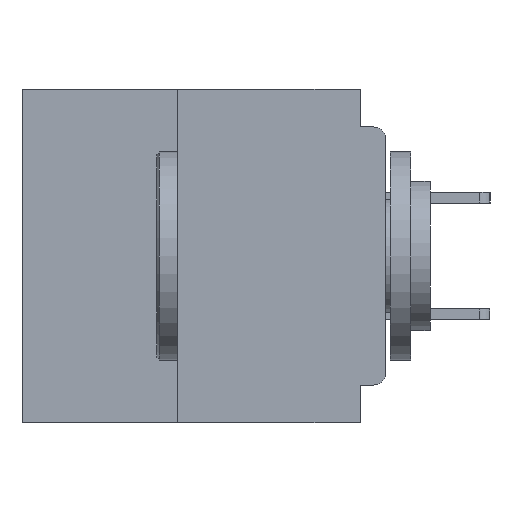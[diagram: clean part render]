
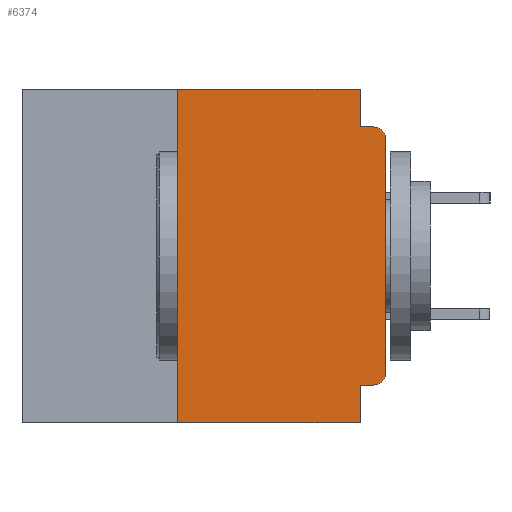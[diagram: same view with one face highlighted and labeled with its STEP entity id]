
A CAD part, left-side view. The second image highlights one B-rep face of the part: STEP entity #6374.
In plain terms, the highlighted planar face has unit normal (-1, 0, 0).
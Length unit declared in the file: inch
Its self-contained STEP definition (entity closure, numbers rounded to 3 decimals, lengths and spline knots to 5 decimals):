
#128 = VECTOR ( 'NONE', #31256, 39.37008 ) ;
#284 = DIRECTION ( 'NONE',  ( -1., 0., 0. ) ) ;
#334 = CARTESIAN_POINT ( 'NONE',  ( 0., 0.031, 0. ) ) ;
#665 = AXIS2_PLACEMENT_3D ( 'NONE', #21856, #284, #25495 ) ;
#1290 = LINE ( 'NONE', #27664, #128 ) ;
#1384 = CIRCLE ( 'NONE', #16615, 0.015 ) ;
#2345 = VERTEX_POINT ( 'NONE', #30027 ) ;
#4031 = LINE ( 'NONE', #44875, #41101 ) ;
#4156 = VERTEX_POINT ( 'NONE', #334 ) ;
#4670 = VECTOR ( 'NONE', #10521, 39.37008 ) ;
#4908 = ORIENTED_EDGE ( 'NONE', *, *, #34543, .T. ) ;
#6158 = VECTOR ( 'NONE', #43915, 39.37008 ) ;
#6374 = ADVANCED_FACE ( 'NONE', ( #24311 ), #21047, .F. ) ;
#6766 = CARTESIAN_POINT ( 'NONE',  ( 0., 0.437, 0. ) ) ;
#7662 = CARTESIAN_POINT ( 'NONE',  ( 0., 0.031, -0.045 ) ) ;
#8150 = EDGE_CURVE ( 'NONE', #38458, #2345, #15741, .T. ) ;
#8468 = CARTESIAN_POINT ( 'NONE',  ( 0., 0.437, -0.4 ) ) ;
#9410 = ORIENTED_EDGE ( 'NONE', *, *, #27634, .T. ) ;
#9823 = VERTEX_POINT ( 'NONE', #33928 ) ;
#10389 = DIRECTION ( 'NONE',  ( 1., 0., 0. ) ) ;
#10521 = DIRECTION ( 'NONE',  ( 0., 0., -1. ) ) ;
#11559 = EDGE_LOOP ( 'NONE', ( #4908, #29991, #24010, #18927, #19372, #18607, #9410, #14994, #15608, #34987 ) ) ;
#11772 = AXIS2_PLACEMENT_3D ( 'NONE', #6766, #10389, #35493 ) ;
#12457 = CARTESIAN_POINT ( 'NONE',  ( 0., 0., -0.06 ) ) ;
#12467 = VERTEX_POINT ( 'NONE', #14058 ) ;
#12930 = EDGE_CURVE ( 'NONE', #43955, #12467, #1290, .T. ) ;
#12963 = DIRECTION ( 'NONE',  ( -1., 0., 0. ) ) ;
#13313 = DIRECTION ( 'NONE',  ( 0., 0., 1. ) ) ;
#14058 = CARTESIAN_POINT ( 'NONE',  ( 0., 0.25, 0. ) ) ;
#14141 = CARTESIAN_POINT ( 'NONE',  ( 0., 0.031, -0.4 ) ) ;
#14639 = EDGE_CURVE ( 'NONE', #4156, #38458, #4031, .T. ) ;
#14994 = ORIENTED_EDGE ( 'NONE', *, *, #24135, .F. ) ;
#15608 = ORIENTED_EDGE ( 'NONE', *, *, #29951, .F. ) ;
#15741 = LINE ( 'NONE', #45934, #23008 ) ;
#16615 = AXIS2_PLACEMENT_3D ( 'NONE', #34432, #12963, #38024 ) ;
#18607 = ORIENTED_EDGE ( 'NONE', *, *, #12930, .F. ) ;
#18927 = ORIENTED_EDGE ( 'NONE', *, *, #14639, .F. ) ;
#19293 = DIRECTION ( 'NONE',  ( 0., -1., 0. ) ) ;
#19372 = ORIENTED_EDGE ( 'NONE', *, *, #29655, .F. ) ;
#21047 = PLANE ( 'NONE',  #11772 ) ;
#21856 = CARTESIAN_POINT ( 'NONE',  ( 0., 0.015, -0.06 ) ) ;
#22746 = VERTEX_POINT ( 'NONE', #37726 ) ;
#22804 = EDGE_CURVE ( 'NONE', #43268, #9823, #1384, .T. ) ;
#23008 = VECTOR ( 'NONE', #28121, 39.37008 ) ;
#23745 = CARTESIAN_POINT ( 'NONE',  ( 0., 0.437, 0. ) ) ;
#23801 = LINE ( 'NONE', #14141, #4670 ) ;
#24010 = ORIENTED_EDGE ( 'NONE', *, *, #8150, .F. ) ;
#24135 = EDGE_CURVE ( 'NONE', #38394, #22746, #23801, .T. ) ;
#24311 = FACE_OUTER_BOUND ( 'NONE', #11559, .T. ) ;
#25262 = LINE ( 'NONE', #33288, #6158 ) ;
#25495 = DIRECTION ( 'NONE',  ( 0., 0., -1. ) ) ;
#27097 = CARTESIAN_POINT ( 'NONE',  ( 0., 0.25, -0.4 ) ) ;
#27634 = EDGE_CURVE ( 'NONE', #43955, #22746, #39466, .T. ) ;
#27664 = CARTESIAN_POINT ( 'NONE',  ( 0., 0.25, -0.4 ) ) ;
#27748 = CARTESIAN_POINT ( 'NONE',  ( 0., 0., 0. ) ) ;
#28121 = DIRECTION ( 'NONE',  ( 0., -1., 0. ) ) ;
#28919 = VERTEX_POINT ( 'NONE', #12457 ) ;
#29655 = EDGE_CURVE ( 'NONE', #12467, #4156, #35374, .T. ) ;
#29951 = EDGE_CURVE ( 'NONE', #43268, #38394, #25262, .T. ) ;
#29991 = ORIENTED_EDGE ( 'NONE', *, *, #33471, .T. ) ;
#30027 = CARTESIAN_POINT ( 'NONE',  ( 0., 0.015, -0.045 ) ) ;
#31256 = DIRECTION ( 'NONE',  ( 0., 0., 1. ) ) ;
#31818 = VECTOR ( 'NONE', #13313, 39.37008 ) ;
#33288 = CARTESIAN_POINT ( 'NONE',  ( 0., 0., -0.355 ) ) ;
#33471 = EDGE_CURVE ( 'NONE', #28919, #2345, #40889, .T. ) ;
#33928 = CARTESIAN_POINT ( 'NONE',  ( 0., 0., -0.34 ) ) ;
#34084 = LINE ( 'NONE', #27748, #31818 ) ;
#34411 = DIRECTION ( 'NONE',  ( 0., -1., 0. ) ) ;
#34432 = CARTESIAN_POINT ( 'NONE',  ( 0., 0.015, -0.34 ) ) ;
#34543 = EDGE_CURVE ( 'NONE', #9823, #28919, #34084, .T. ) ;
#34987 = ORIENTED_EDGE ( 'NONE', *, *, #22804, .T. ) ;
#35374 = LINE ( 'NONE', #23745, #44868 ) ;
#35493 = DIRECTION ( 'NONE',  ( 0., 0., -1. ) ) ;
#37726 = CARTESIAN_POINT ( 'NONE',  ( 0., 0.031, -0.4 ) ) ;
#38024 = DIRECTION ( 'NONE',  ( 0., 0., -1. ) ) ;
#38362 = VECTOR ( 'NONE', #19293, 39.37008 ) ;
#38394 = VERTEX_POINT ( 'NONE', #43063 ) ;
#38458 = VERTEX_POINT ( 'NONE', #7662 ) ;
#39466 = LINE ( 'NONE', #8468, #38362 ) ;
#40889 = CIRCLE ( 'NONE', #665, 0.015 ) ;
#41101 = VECTOR ( 'NONE', #42266, 39.37008 ) ;
#42266 = DIRECTION ( 'NONE',  ( 0., 0., -1. ) ) ;
#42933 = CARTESIAN_POINT ( 'NONE',  ( 0., 0.015, -0.355 ) ) ;
#43063 = CARTESIAN_POINT ( 'NONE',  ( 0., 0.031, -0.355 ) ) ;
#43268 = VERTEX_POINT ( 'NONE', #42933 ) ;
#43915 = DIRECTION ( 'NONE',  ( 0., 1., 0. ) ) ;
#43955 = VERTEX_POINT ( 'NONE', #27097 ) ;
#44868 = VECTOR ( 'NONE', #34411, 39.37008 ) ;
#44875 = CARTESIAN_POINT ( 'NONE',  ( 0., 0.031, 0. ) ) ;
#45934 = CARTESIAN_POINT ( 'NONE',  ( 0., 0., -0.045 ) ) ;
